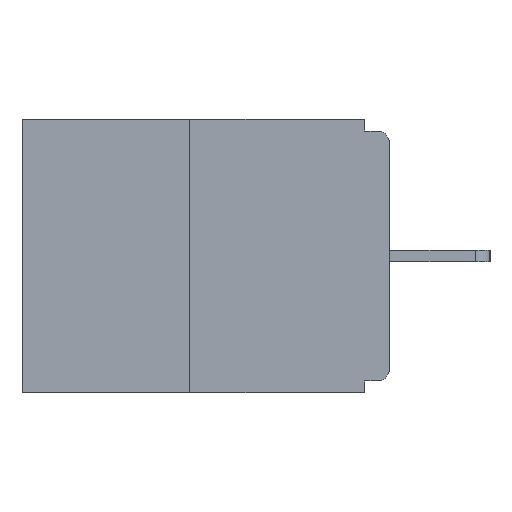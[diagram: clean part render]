
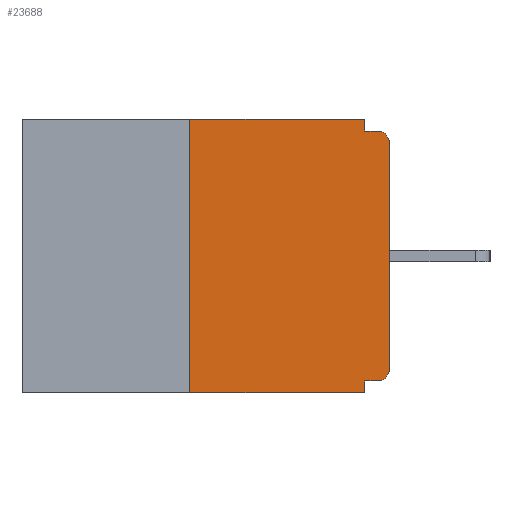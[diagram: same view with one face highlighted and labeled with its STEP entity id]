
A CAD part, left-side view. The second image highlights one B-rep face of the part: STEP entity #23688.
In plain terms, the highlighted planar face has unit normal (-1, 0, 0).
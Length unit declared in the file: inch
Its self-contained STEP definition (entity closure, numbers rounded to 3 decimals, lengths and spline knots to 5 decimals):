
#7 = EDGE_CURVE ( 'NONE', #25296, #7197, #24559, .T. ) ;
#542 = DIRECTION ( 'NONE',  ( 0., 0., 1. ) ) ;
#596 = DIRECTION ( 'NONE',  ( 0., -1., 0. ) ) ;
#822 = VECTOR ( 'NONE', #12997, 39.37008 ) ;
#1560 = LINE ( 'NONE', #27902, #822 ) ;
#2081 = VECTOR ( 'NONE', #596, 39.37008 ) ;
#2159 = ORIENTED_EDGE ( 'NONE', *, *, #26210, .F. ) ;
#2320 = AXIS2_PLACEMENT_3D ( 'NONE', #25955, #19559, #6544 ) ;
#2486 = EDGE_CURVE ( 'NONE', #22140, #25296, #1560, .T. ) ;
#2623 = AXIS2_PLACEMENT_3D ( 'NONE', #9895, #25094, #12069 ) ;
#3072 = CARTESIAN_POINT ( 'NONE',  ( 0., 0.25, -0.343 ) ) ;
#3610 = CARTESIAN_POINT ( 'NONE',  ( 0., 0.031, -0.015 ) ) ;
#4234 = EDGE_CURVE ( 'NONE', #4694, #20267, #15283, .T. ) ;
#4694 = VERTEX_POINT ( 'NONE', #10712 ) ;
#5020 = DIRECTION ( 'NONE',  ( 0., -1., 0. ) ) ;
#6001 = ORIENTED_EDGE ( 'NONE', *, *, #2486, .F. ) ;
#6143 = CARTESIAN_POINT ( 'NONE',  ( 0., 0.031, -0.343 ) ) ;
#6285 = CARTESIAN_POINT ( 'NONE',  ( 0., 0.015, -0.03 ) ) ;
#6544 = DIRECTION ( 'NONE',  ( 0., 0., -1. ) ) ;
#7197 = VERTEX_POINT ( 'NONE', #17680 ) ;
#7556 = CARTESIAN_POINT ( 'NONE',  ( 0., 0.015, -0.328 ) ) ;
#8617 = LINE ( 'NONE', #11566, #2081 ) ;
#8858 = EDGE_CURVE ( 'NONE', #11840, #20267, #8617, .T. ) ;
#9026 = ORIENTED_EDGE ( 'NONE', *, *, #13463, .F. ) ;
#9260 = CARTESIAN_POINT ( 'NONE',  ( 0., 0.46, 0. ) ) ;
#9438 = EDGE_CURVE ( 'NONE', #27027, #27304, #14655, .T. ) ;
#9689 = ORIENTED_EDGE ( 'NONE', *, *, #9438, .F. ) ;
#9895 = CARTESIAN_POINT ( 'NONE',  ( 0., 0.015, -0.313 ) ) ;
#10132 = LINE ( 'NONE', #10815, #26746 ) ;
#10170 = EDGE_CURVE ( 'NONE', #22140, #13018, #15457, .T. ) ;
#10712 = CARTESIAN_POINT ( 'NONE',  ( 0., 0., -0.03 ) ) ;
#10815 = CARTESIAN_POINT ( 'NONE',  ( 0., 0.031, 0. ) ) ;
#11566 = CARTESIAN_POINT ( 'NONE',  ( 0., 0., -0.015 ) ) ;
#11636 = CARTESIAN_POINT ( 'NONE',  ( 0., 0.46, -0.343 ) ) ;
#11726 = ORIENTED_EDGE ( 'NONE', *, *, #10170, .T. ) ;
#11840 = VERTEX_POINT ( 'NONE', #3610 ) ;
#12069 = DIRECTION ( 'NONE',  ( 0., 0., -1. ) ) ;
#12997 = DIRECTION ( 'NONE',  ( 0., 1., 0. ) ) ;
#13018 = VERTEX_POINT ( 'NONE', #22993 ) ;
#13246 = VECTOR ( 'NONE', #5020, 39.37008 ) ;
#13463 = EDGE_CURVE ( 'NONE', #27304, #26265, #19086, .T. ) ;
#13972 = VECTOR ( 'NONE', #17928, 39.37008 ) ;
#14655 = LINE ( 'NONE', #15624, #13972 ) ;
#15283 = CIRCLE ( 'NONE', #16869, 0.015 ) ;
#15457 = CIRCLE ( 'NONE', #2623, 0.015 ) ;
#15460 = ORIENTED_EDGE ( 'NONE', *, *, #23330, .T. ) ;
#15624 = CARTESIAN_POINT ( 'NONE',  ( 0., 0.25, 0. ) ) ;
#15769 = CARTESIAN_POINT ( 'NONE',  ( 0., 0.031, 0. ) ) ;
#16005 = DIRECTION ( 'NONE',  ( 0., -1., 0. ) ) ;
#16869 = AXIS2_PLACEMENT_3D ( 'NONE', #6285, #22006, #21940 ) ;
#17038 = DIRECTION ( 'NONE',  ( 0., 0., -1. ) ) ;
#17320 = PLANE ( 'NONE',  #2320 ) ;
#17432 = LINE ( 'NONE', #26688, #28228 ) ;
#17680 = CARTESIAN_POINT ( 'NONE',  ( 0., 0.031, -0.343 ) ) ;
#17928 = DIRECTION ( 'NONE',  ( 0., 0., 1. ) ) ;
#18231 = ORIENTED_EDGE ( 'NONE', *, *, #20291, .T. ) ;
#19086 = LINE ( 'NONE', #9260, #13246 ) ;
#19559 = DIRECTION ( 'NONE',  ( 1., 0., 0. ) ) ;
#20131 = CARTESIAN_POINT ( 'NONE',  ( 0., 0.015, -0.015 ) ) ;
#20267 = VERTEX_POINT ( 'NONE', #20131 ) ;
#20291 = EDGE_CURVE ( 'NONE', #13018, #4694, #17432, .T. ) ;
#21471 = CARTESIAN_POINT ( 'NONE',  ( 0., 0.25, 0. ) ) ;
#21940 = DIRECTION ( 'NONE',  ( 0., 0., -1. ) ) ;
#21967 = ORIENTED_EDGE ( 'NONE', *, *, #7, .F. ) ;
#22006 = DIRECTION ( 'NONE',  ( -1., 0., 0. ) ) ;
#22140 = VERTEX_POINT ( 'NONE', #7556 ) ;
#22237 = EDGE_LOOP ( 'NONE', ( #9026, #9689, #15460, #21967, #6001, #11726, #18231, #23995, #24660, #2159 ) ) ;
#22993 = CARTESIAN_POINT ( 'NONE',  ( 0., 0., -0.313 ) ) ;
#23075 = CARTESIAN_POINT ( 'NONE',  ( 0., 0.031, -0.328 ) ) ;
#23330 = EDGE_CURVE ( 'NONE', #27027, #7197, #24937, .T. ) ;
#23688 = ADVANCED_FACE ( 'NONE', ( #26241 ), #17320, .F. ) ;
#23881 = DIRECTION ( 'NONE',  ( 0., 0., -1. ) ) ;
#23888 = VECTOR ( 'NONE', #17038, 39.37008 ) ;
#23995 = ORIENTED_EDGE ( 'NONE', *, *, #4234, .T. ) ;
#24275 = VECTOR ( 'NONE', #16005, 39.37008 ) ;
#24559 = LINE ( 'NONE', #6143, #23888 ) ;
#24660 = ORIENTED_EDGE ( 'NONE', *, *, #8858, .F. ) ;
#24937 = LINE ( 'NONE', #11636, #24275 ) ;
#25094 = DIRECTION ( 'NONE',  ( -1., 0., 0. ) ) ;
#25296 = VERTEX_POINT ( 'NONE', #23075 ) ;
#25955 = CARTESIAN_POINT ( 'NONE',  ( 0., 0.46, 0. ) ) ;
#26210 = EDGE_CURVE ( 'NONE', #26265, #11840, #10132, .T. ) ;
#26241 = FACE_OUTER_BOUND ( 'NONE', #22237, .T. ) ;
#26265 = VERTEX_POINT ( 'NONE', #15769 ) ;
#26688 = CARTESIAN_POINT ( 'NONE',  ( 0., 0., 0. ) ) ;
#26746 = VECTOR ( 'NONE', #23881, 39.37008 ) ;
#27027 = VERTEX_POINT ( 'NONE', #3072 ) ;
#27304 = VERTEX_POINT ( 'NONE', #21471 ) ;
#27902 = CARTESIAN_POINT ( 'NONE',  ( 0., 0., -0.328 ) ) ;
#28228 = VECTOR ( 'NONE', #542, 39.37008 ) ;
